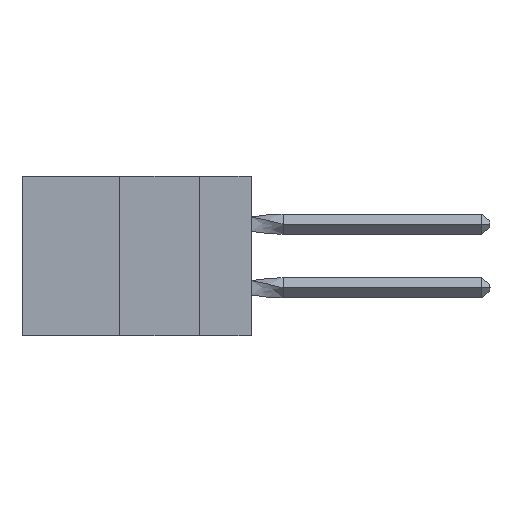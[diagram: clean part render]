
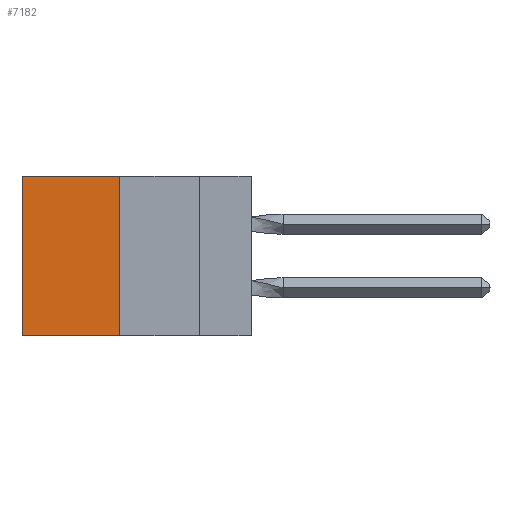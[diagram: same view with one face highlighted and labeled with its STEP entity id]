
A CAD part, left-side view. The second image highlights one B-rep face of the part: STEP entity #7182.
In plain terms, the highlighted planar face has unit normal (-1, 0, 0).
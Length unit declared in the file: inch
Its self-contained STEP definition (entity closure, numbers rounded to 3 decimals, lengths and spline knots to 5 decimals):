
#354 = LINE ( 'NONE', #26725, #2596 ) ;
#1680 = EDGE_CURVE ( 'NONE', #14084, #22696, #27226, .T. ) ;
#2596 = VECTOR ( 'NONE', #17432, 39.37008 ) ;
#2926 = ORIENTED_EDGE ( 'NONE', *, *, #1680, .T. ) ;
#4184 = VERTEX_POINT ( 'NONE', #7484 ) ;
#6451 = PLANE ( 'NONE',  #10065 ) ;
#6852 = VECTOR ( 'NONE', #29084, 39.37008 ) ;
#7182 = ADVANCED_FACE ( 'NONE', ( #27600 ), #6451, .F. ) ;
#7484 = CARTESIAN_POINT ( 'NONE',  ( 0.305, 0.72, -0.5 ) ) ;
#7800 = CARTESIAN_POINT ( 'NONE',  ( 0.305, 0.413, 0. ) ) ;
#10065 = AXIS2_PLACEMENT_3D ( 'NONE', #11223, #23086, #25576 ) ;
#11180 = CARTESIAN_POINT ( 'NONE',  ( 0.305, 0.413, 0. ) ) ;
#11223 = CARTESIAN_POINT ( 'NONE',  ( 0.305, 0.413, -0.5 ) ) ;
#11782 = ORIENTED_EDGE ( 'NONE', *, *, #26293, .T. ) ;
#12094 = LINE ( 'NONE', #15210, #27246 ) ;
#12929 = VECTOR ( 'NONE', #21148, 39.37008 ) ;
#13742 = EDGE_CURVE ( 'NONE', #14084, #25357, #354, .T. ) ;
#14010 = CARTESIAN_POINT ( 'NONE',  ( 0.305, 0.413, -0.5 ) ) ;
#14084 = VERTEX_POINT ( 'NONE', #11180 ) ;
#15210 = CARTESIAN_POINT ( 'NONE',  ( 0.305, 0.72, -0.5 ) ) ;
#17432 = DIRECTION ( 'NONE',  ( 0., 0., -1. ) ) ;
#18666 = EDGE_LOOP ( 'NONE', ( #11782, #25157, #29719, #2926 ) ) ;
#20012 = DIRECTION ( 'NONE',  ( 0., 0., -1. ) ) ;
#21148 = DIRECTION ( 'NONE',  ( 0., 1., 0. ) ) ;
#22696 = VERTEX_POINT ( 'NONE', #27418 ) ;
#23086 = DIRECTION ( 'NONE',  ( 1., 0., 0. ) ) ;
#23210 = CARTESIAN_POINT ( 'NONE',  ( 0.305, 0.413, -0.5 ) ) ;
#23615 = EDGE_CURVE ( 'NONE', #25357, #4184, #27692, .T. ) ;
#25157 = ORIENTED_EDGE ( 'NONE', *, *, #23615, .F. ) ;
#25357 = VERTEX_POINT ( 'NONE', #14010 ) ;
#25576 = DIRECTION ( 'NONE',  ( 0., 0., -1. ) ) ;
#26293 = EDGE_CURVE ( 'NONE', #22696, #4184, #12094, .T. ) ;
#26725 = CARTESIAN_POINT ( 'NONE',  ( 0.305, 0.413, -0.5 ) ) ;
#27226 = LINE ( 'NONE', #7800, #6852 ) ;
#27246 = VECTOR ( 'NONE', #20012, 39.37008 ) ;
#27418 = CARTESIAN_POINT ( 'NONE',  ( 0.305, 0.72, 0. ) ) ;
#27600 = FACE_OUTER_BOUND ( 'NONE', #18666, .T. ) ;
#27692 = LINE ( 'NONE', #23210, #12929 ) ;
#29084 = DIRECTION ( 'NONE',  ( 0., 1., 0. ) ) ;
#29719 = ORIENTED_EDGE ( 'NONE', *, *, #13742, .F. ) ;
